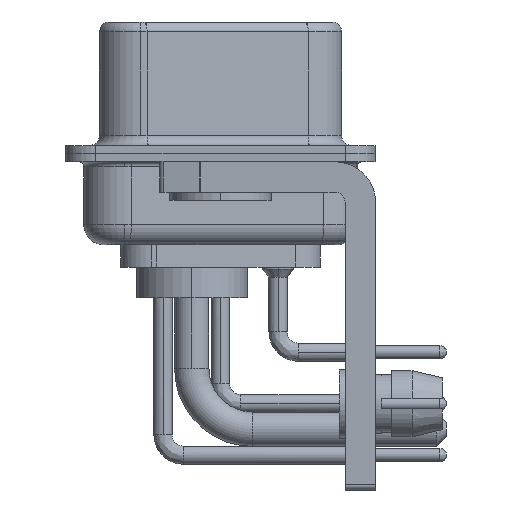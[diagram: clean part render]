
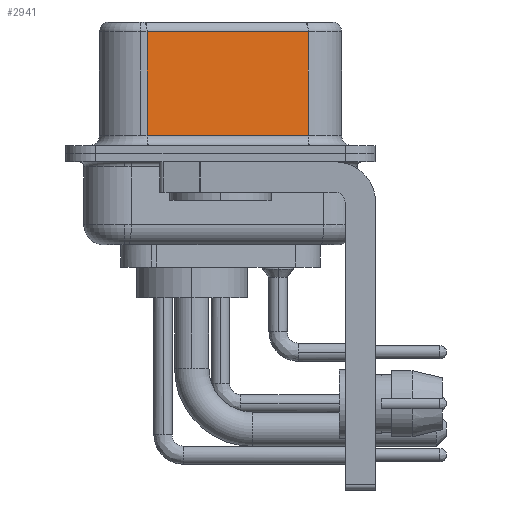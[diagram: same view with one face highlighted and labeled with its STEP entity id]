
A CAD part, left-side view. The second image highlights one B-rep face of the part: STEP entity #2941.
In plain terms, the highlighted planar face has unit normal (-0.985, -0.174, 0).
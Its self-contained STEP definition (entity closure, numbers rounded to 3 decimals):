
#794 = EDGE_LOOP ( 'NONE', ( #1149, #21772, #22075, #18578 ) ) ;
#950 = VERTEX_POINT ( 'NONE', #34014 ) ;
#1149 = ORIENTED_EDGE ( 'NONE', *, *, #6871, .F. ) ;
#1842 = VECTOR ( 'NONE', #23093, 1000. ) ;
#1938 = EDGE_CURVE ( 'NONE', #17056, #22476, #26538, .T. ) ;
#2802 = CARTESIAN_POINT ( 'NONE',  ( 3.73, 3.628, 6.52 ) ) ;
#2941 = ADVANCED_FACE ( 'NONE', ( #3325 ), #9234, .F. ) ;
#3325 = FACE_OUTER_BOUND ( 'NONE', #794, .T. ) ;
#6185 = CARTESIAN_POINT ( 'NONE',  ( 5.132, -4.322, 6.02 ) ) ;
#6871 = EDGE_CURVE ( 'NONE', #17056, #31226, #30196, .T. ) ;
#6950 = EDGE_CURVE ( 'NONE', #22476, #950, #16883, .T. ) ;
#9234 = PLANE ( 'NONE',  #12554 ) ;
#9826 = CARTESIAN_POINT ( 'NONE',  ( 5.132, -4.322, 0.9 ) ) ;
#9854 = DIRECTION ( 'NONE',  ( -0.174, 0.985, 0. ) ) ;
#11472 = VECTOR ( 'NONE', #17032, 1000. ) ;
#11478 = CARTESIAN_POINT ( 'NONE',  ( 5.132, -4.322, 0.9 ) ) ;
#11826 = DIRECTION ( 'NONE',  ( 0.985, 0.174, 0. ) ) ;
#12316 = VECTOR ( 'NONE', #9854, 1000. ) ;
#12554 = AXIS2_PLACEMENT_3D ( 'NONE', #23108, #11826, #34441 ) ;
#13658 = CARTESIAN_POINT ( 'NONE',  ( 3.73, 3.628, 6.02 ) ) ;
#16883 = LINE ( 'NONE', #2802, #26125 ) ;
#17032 = DIRECTION ( 'NONE',  ( 0.174, -0.985, 0. ) ) ;
#17056 = VERTEX_POINT ( 'NONE', #18722 ) ;
#18578 = ORIENTED_EDGE ( 'NONE', *, *, #28954, .T. ) ;
#18722 = CARTESIAN_POINT ( 'NONE',  ( 5.132, -4.322, 6.02 ) ) ;
#21772 = ORIENTED_EDGE ( 'NONE', *, *, #1938, .T. ) ;
#22075 = ORIENTED_EDGE ( 'NONE', *, *, #6950, .T. ) ;
#22476 = VERTEX_POINT ( 'NONE', #13658 ) ;
#23093 = DIRECTION ( 'NONE',  ( 0., 0., -1. ) ) ;
#23108 = CARTESIAN_POINT ( 'NONE',  ( 5.132, -4.322, 6.52 ) ) ;
#25890 = DIRECTION ( 'NONE',  ( 0., 0., -1. ) ) ;
#26125 = VECTOR ( 'NONE', #25890, 1000. ) ;
#26538 = LINE ( 'NONE', #6185, #12316 ) ;
#28181 = CARTESIAN_POINT ( 'NONE',  ( 5.132, -4.322, 6.52 ) ) ;
#28954 = EDGE_CURVE ( 'NONE', #950, #31226, #30365, .T. ) ;
#30196 = LINE ( 'NONE', #28181, #1842 ) ;
#30365 = LINE ( 'NONE', #11478, #11472 ) ;
#31226 = VERTEX_POINT ( 'NONE', #9826 ) ;
#34014 = CARTESIAN_POINT ( 'NONE',  ( 3.73, 3.628, 0.9 ) ) ;
#34441 = DIRECTION ( 'NONE',  ( -0.174, 0.985, 0. ) ) ;
